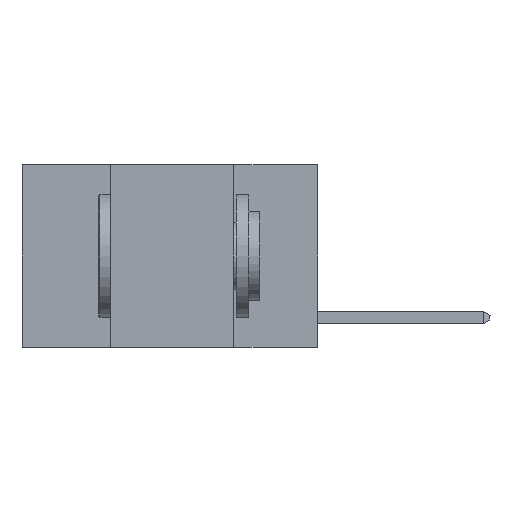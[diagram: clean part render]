
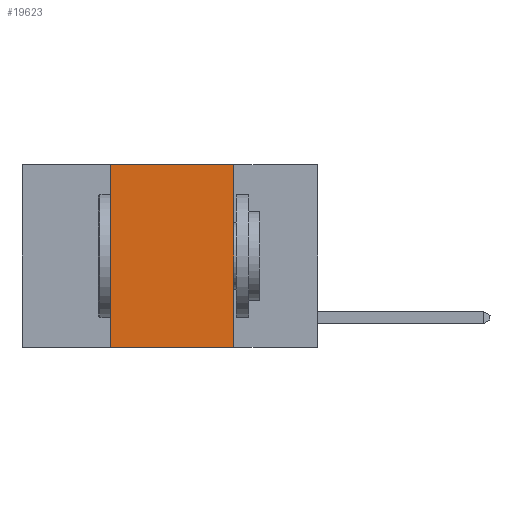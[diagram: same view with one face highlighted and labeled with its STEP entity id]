
A CAD part, left-side view. The second image highlights one B-rep face of the part: STEP entity #19623.
In plain terms, the highlighted planar face has unit normal (-1, 0, 0).
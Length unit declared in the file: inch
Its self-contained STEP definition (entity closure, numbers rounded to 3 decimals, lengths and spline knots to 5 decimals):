
#301 = ORIENTED_EDGE ( 'NONE', *, *, #22514, .F. ) ;
#374 = VECTOR ( 'NONE', #19401, 39.37008 ) ;
#542 = DIRECTION ( 'NONE',  ( 0., -1., 0. ) ) ;
#2894 = LINE ( 'NONE', #22951, #374 ) ;
#4180 = EDGE_CURVE ( 'NONE', #20423, #22890, #19821, .T. ) ;
#6524 = CARTESIAN_POINT ( 'NONE',  ( 0., 0.17, 0. ) ) ;
#6973 = DIRECTION ( 'NONE',  ( 1., 0., 0. ) ) ;
#9695 = DIRECTION ( 'NONE',  ( 0., -1., 0. ) ) ;
#10136 = CARTESIAN_POINT ( 'NONE',  ( 0., 0.17, -0.37 ) ) ;
#10982 = VECTOR ( 'NONE', #9695, 39.37008 ) ;
#11123 = DIRECTION ( 'NONE',  ( 0., 0., -1. ) ) ;
#11147 = VERTEX_POINT ( 'NONE', #21642 ) ;
#11275 = ORIENTED_EDGE ( 'NONE', *, *, #18422, .F. ) ;
#11375 = EDGE_CURVE ( 'NONE', #11147, #16265, #24100, .T. ) ;
#12195 = EDGE_LOOP ( 'NONE', ( #301, #19459, #11275, #18799 ) ) ;
#13137 = VECTOR ( 'NONE', #11123, 39.37008 ) ;
#14852 = DIRECTION ( 'NONE',  ( 0., 0., -1. ) ) ;
#15112 = CARTESIAN_POINT ( 'NONE',  ( 0., 0.6, 0. ) ) ;
#15499 = CARTESIAN_POINT ( 'NONE',  ( 0., 0.6, 0. ) ) ;
#16265 = VERTEX_POINT ( 'NONE', #10136 ) ;
#16357 = CARTESIAN_POINT ( 'NONE',  ( 0., 0.42, 0. ) ) ;
#17171 = LINE ( 'NONE', #24986, #13137 ) ;
#18422 = EDGE_CURVE ( 'NONE', #11147, #20423, #2894, .T. ) ;
#18799 = ORIENTED_EDGE ( 'NONE', *, *, #11375, .T. ) ;
#18939 = FACE_OUTER_BOUND ( 'NONE', #12195, .T. ) ;
#19401 = DIRECTION ( 'NONE',  ( 0., 0., 1. ) ) ;
#19459 = ORIENTED_EDGE ( 'NONE', *, *, #4180, .F. ) ;
#19623 = ADVANCED_FACE ( 'NONE', ( #18939 ), #24776, .F. ) ;
#19821 = LINE ( 'NONE', #15499, #10982 ) ;
#20423 = VERTEX_POINT ( 'NONE', #16357 ) ;
#21642 = CARTESIAN_POINT ( 'NONE',  ( 0., 0.42, -0.37 ) ) ;
#21681 = VECTOR ( 'NONE', #542, 39.37008 ) ;
#22034 = CARTESIAN_POINT ( 'NONE',  ( 0., 0.6, -0.37 ) ) ;
#22514 = EDGE_CURVE ( 'NONE', #22890, #16265, #17171, .T. ) ;
#22890 = VERTEX_POINT ( 'NONE', #6524 ) ;
#22951 = CARTESIAN_POINT ( 'NONE',  ( 0., 0.42, 0. ) ) ;
#24100 = LINE ( 'NONE', #22034, #21681 ) ;
#24776 = PLANE ( 'NONE',  #25512 ) ;
#24986 = CARTESIAN_POINT ( 'NONE',  ( 0., 0.17, 0. ) ) ;
#25512 = AXIS2_PLACEMENT_3D ( 'NONE', #15112, #6973, #14852 ) ;
